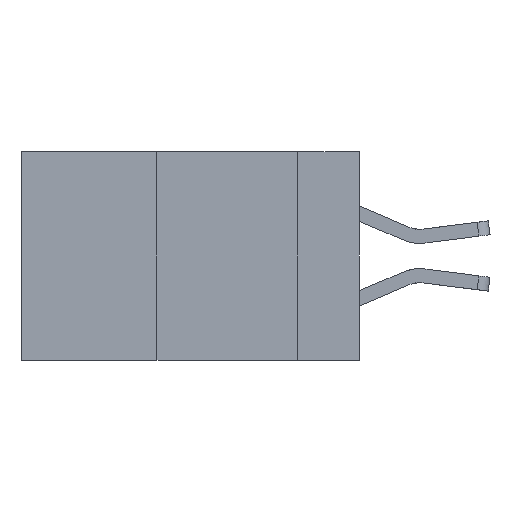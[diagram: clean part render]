
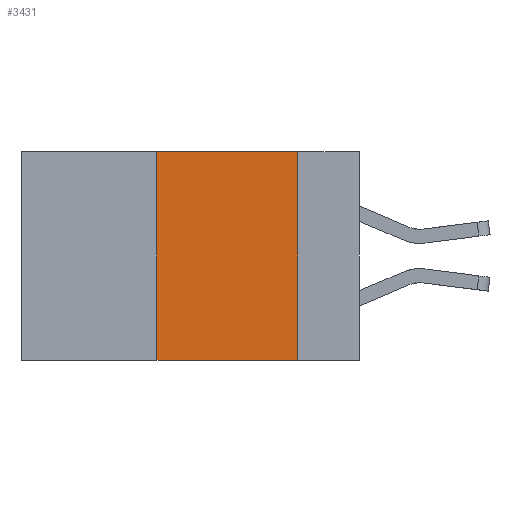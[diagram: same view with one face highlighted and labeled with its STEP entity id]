
A CAD part, left-side view. The second image highlights one B-rep face of the part: STEP entity #3431.
In plain terms, the highlighted planar face has unit normal (-1, 0, 0).
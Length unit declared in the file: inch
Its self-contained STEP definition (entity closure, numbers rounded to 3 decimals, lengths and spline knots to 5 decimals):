
#244 = VECTOR ( 'NONE', #5626, 39.37008 ) ;
#481 = VECTOR ( 'NONE', #2808, 39.37008 ) ;
#609 = CARTESIAN_POINT ( 'NONE',  ( 0., 0.36, 0. ) ) ;
#1326 = CARTESIAN_POINT ( 'NONE',  ( 0., 0.11, 0. ) ) ;
#2196 = DIRECTION ( 'NONE',  ( 1., 0., 0. ) ) ;
#2704 = EDGE_LOOP ( 'NONE', ( #11753, #5749, #9034, #6115 ) ) ;
#2767 = CARTESIAN_POINT ( 'NONE',  ( 0., 0.36, 0. ) ) ;
#2808 = DIRECTION ( 'NONE',  ( 0., 0., 1. ) ) ;
#3391 = LINE ( 'NONE', #4367, #244 ) ;
#3431 = ADVANCED_FACE ( 'NONE', ( #6865 ), #3522, .F. ) ;
#3522 = PLANE ( 'NONE',  #14270 ) ;
#3588 = LINE ( 'NONE', #2767, #481 ) ;
#3748 = CARTESIAN_POINT ( 'NONE',  ( 0., 0.36, -0.37 ) ) ;
#4335 = EDGE_CURVE ( 'NONE', #11901, #4723, #3588, .T. ) ;
#4367 = CARTESIAN_POINT ( 'NONE',  ( 0., 0.6, -0.37 ) ) ;
#4567 = VECTOR ( 'NONE', #7314, 39.37008 ) ;
#4723 = VERTEX_POINT ( 'NONE', #609 ) ;
#4845 = CARTESIAN_POINT ( 'NONE',  ( 0., 0.6, 0. ) ) ;
#5133 = EDGE_CURVE ( 'NONE', #7284, #11120, #13174, .T. ) ;
#5626 = DIRECTION ( 'NONE',  ( 0., -1., 0. ) ) ;
#5749 = ORIENTED_EDGE ( 'NONE', *, *, #11194, .F. ) ;
#6115 = ORIENTED_EDGE ( 'NONE', *, *, #6790, .T. ) ;
#6692 = CARTESIAN_POINT ( 'NONE',  ( 0., 0.11, 0. ) ) ;
#6790 = EDGE_CURVE ( 'NONE', #11901, #11120, #3391, .T. ) ;
#6865 = FACE_OUTER_BOUND ( 'NONE', #2704, .T. ) ;
#7010 = VECTOR ( 'NONE', #9699, 39.37008 ) ;
#7284 = VERTEX_POINT ( 'NONE', #6692 ) ;
#7314 = DIRECTION ( 'NONE',  ( 0., -1., 0. ) ) ;
#7843 = LINE ( 'NONE', #4845, #4567 ) ;
#8425 = DIRECTION ( 'NONE',  ( 0., 0., -1. ) ) ;
#9034 = ORIENTED_EDGE ( 'NONE', *, *, #4335, .F. ) ;
#9664 = CARTESIAN_POINT ( 'NONE',  ( 0., 0.11, -0.37 ) ) ;
#9699 = DIRECTION ( 'NONE',  ( 0., 0., -1. ) ) ;
#10790 = CARTESIAN_POINT ( 'NONE',  ( 0., 0.6, 0. ) ) ;
#11120 = VERTEX_POINT ( 'NONE', #9664 ) ;
#11194 = EDGE_CURVE ( 'NONE', #4723, #7284, #7843, .T. ) ;
#11753 = ORIENTED_EDGE ( 'NONE', *, *, #5133, .F. ) ;
#11901 = VERTEX_POINT ( 'NONE', #3748 ) ;
#13174 = LINE ( 'NONE', #1326, #7010 ) ;
#14270 = AXIS2_PLACEMENT_3D ( 'NONE', #10790, #2196, #8425 ) ;
